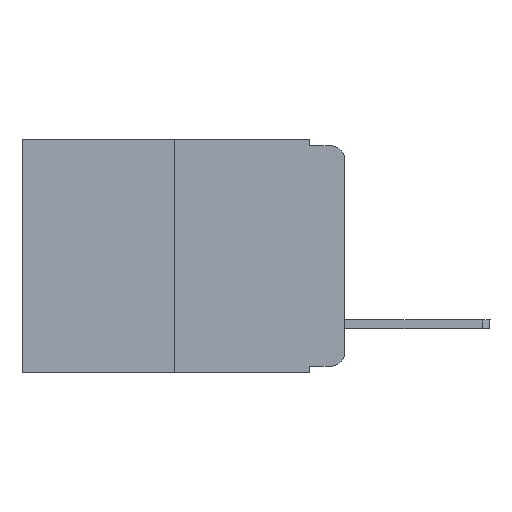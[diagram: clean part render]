
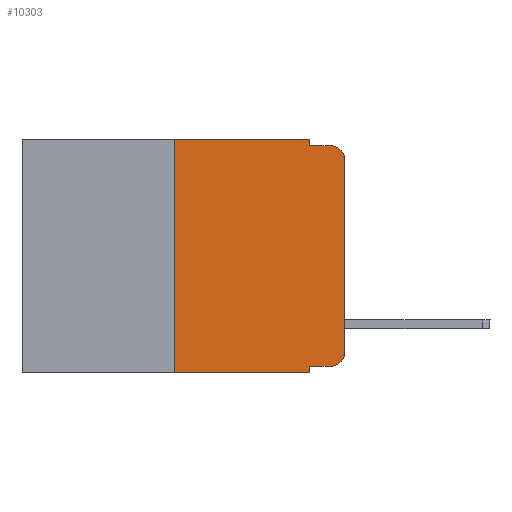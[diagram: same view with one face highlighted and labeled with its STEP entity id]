
A CAD part, left-side view. The second image highlights one B-rep face of the part: STEP entity #10303.
In plain terms, the highlighted planar face has unit normal (-1, 0, 0).
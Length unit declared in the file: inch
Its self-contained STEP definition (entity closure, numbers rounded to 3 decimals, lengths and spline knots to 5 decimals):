
#290 = VECTOR ( 'NONE', #5086, 39.37008 ) ;
#769 = CIRCLE ( 'NONE', #4019, 0.02 ) ;
#863 = ORIENTED_EDGE ( 'NONE', *, *, #11971, .T. ) ;
#1033 = ORIENTED_EDGE ( 'NONE', *, *, #11320, .F. ) ;
#1575 = VERTEX_POINT ( 'NONE', #14547 ) ;
#1820 = CARTESIAN_POINT ( 'NONE',  ( 0., 0.473, -0.343 ) ) ;
#1895 = LINE ( 'NONE', #1820, #14718 ) ;
#1922 = VERTEX_POINT ( 'NONE', #6890 ) ;
#2300 = EDGE_CURVE ( 'NONE', #1575, #3261, #2522, .T. ) ;
#2522 = LINE ( 'NONE', #7733, #9561 ) ;
#2606 = ORIENTED_EDGE ( 'NONE', *, *, #13235, .F. ) ;
#2616 = CARTESIAN_POINT ( 'NONE',  ( 0., 0.02, -0.313 ) ) ;
#2626 = LINE ( 'NONE', #11511, #290 ) ;
#2684 = EDGE_LOOP ( 'NONE', ( #15539, #863, #11656, #2606, #13786, #15054, #15966, #1033, #13511, #13650 ) ) ;
#2707 = CIRCLE ( 'NONE', #13351, 0.02 ) ;
#3261 = VERTEX_POINT ( 'NONE', #16416 ) ;
#3397 = VECTOR ( 'NONE', #13027, 39.37008 ) ;
#3613 = CARTESIAN_POINT ( 'NONE',  ( 0., 0., -0.03 ) ) ;
#3797 = PLANE ( 'NONE',  #15312 ) ;
#4019 = AXIS2_PLACEMENT_3D ( 'NONE', #2616, #7643, #11749 ) ;
#4460 = CARTESIAN_POINT ( 'NONE',  ( 0., 0.051, -0.343 ) ) ;
#4523 = VERTEX_POINT ( 'NONE', #6047 ) ;
#4895 = VERTEX_POINT ( 'NONE', #15977 ) ;
#5086 = DIRECTION ( 'NONE',  ( 0., 0., -1. ) ) ;
#5501 = EDGE_CURVE ( 'NONE', #10545, #11699, #16624, .T. ) ;
#5786 = VECTOR ( 'NONE', #5889, 39.37008 ) ;
#5889 = DIRECTION ( 'NONE',  ( 0., 0., -1. ) ) ;
#6047 = CARTESIAN_POINT ( 'NONE',  ( 0., 0.051, -0.01 ) ) ;
#6185 = CARTESIAN_POINT ( 'NONE',  ( 0., 0.25, 0. ) ) ;
#6357 = DIRECTION ( 'NONE',  ( 1., 0., 0. ) ) ;
#6890 = CARTESIAN_POINT ( 'NONE',  ( 0., 0., -0.313 ) ) ;
#7018 = DIRECTION ( 'NONE',  ( 0., -1., 0. ) ) ;
#7461 = CARTESIAN_POINT ( 'NONE',  ( 0., 0.051, -0.333 ) ) ;
#7544 = CARTESIAN_POINT ( 'NONE',  ( 0., 0.25, -0.343 ) ) ;
#7566 = LINE ( 'NONE', #6185, #9086 ) ;
#7643 = DIRECTION ( 'NONE',  ( -1., 0., 0. ) ) ;
#7645 = FACE_OUTER_BOUND ( 'NONE', #2684, .T. ) ;
#7733 = CARTESIAN_POINT ( 'NONE',  ( 0., 0.473, 0. ) ) ;
#8973 = EDGE_CURVE ( 'NONE', #11699, #1922, #769, .T. ) ;
#9086 = VECTOR ( 'NONE', #10475, 39.37008 ) ;
#9307 = CARTESIAN_POINT ( 'NONE',  ( 0., 0.051, -0.01 ) ) ;
#9561 = VECTOR ( 'NONE', #12958, 39.37008 ) ;
#9745 = EDGE_CURVE ( 'NONE', #16707, #12029, #1895, .T. ) ;
#10303 = ADVANCED_FACE ( 'NONE', ( #7645 ), #3797, .F. ) ;
#10361 = CARTESIAN_POINT ( 'NONE',  ( 0., 0.051, -0.333 ) ) ;
#10475 = DIRECTION ( 'NONE',  ( 0., 0., 1. ) ) ;
#10545 = VERTEX_POINT ( 'NONE', #7461 ) ;
#10773 = DIRECTION ( 'NONE',  ( 0., -1., 0. ) ) ;
#10793 = VECTOR ( 'NONE', #12101, 39.37008 ) ;
#10930 = LINE ( 'NONE', #9307, #14255 ) ;
#11320 = EDGE_CURVE ( 'NONE', #10545, #12029, #16822, .T. ) ;
#11468 = EDGE_CURVE ( 'NONE', #1922, #16649, #12011, .T. ) ;
#11511 = CARTESIAN_POINT ( 'NONE',  ( 0., 0.051, 0. ) ) ;
#11588 = DIRECTION ( 'NONE',  ( 0., 0., -1. ) ) ;
#11656 = ORIENTED_EDGE ( 'NONE', *, *, #15476, .F. ) ;
#11699 = VERTEX_POINT ( 'NONE', #13806 ) ;
#11749 = DIRECTION ( 'NONE',  ( 0., 0., -1. ) ) ;
#11971 = EDGE_CURVE ( 'NONE', #16649, #4895, #2707, .T. ) ;
#12011 = LINE ( 'NONE', #15859, #10793 ) ;
#12029 = VERTEX_POINT ( 'NONE', #4460 ) ;
#12101 = DIRECTION ( 'NONE',  ( 0., 0., 1. ) ) ;
#12869 = CARTESIAN_POINT ( 'NONE',  ( 0., 0.473, 0. ) ) ;
#12958 = DIRECTION ( 'NONE',  ( 0., -1., 0. ) ) ;
#13027 = DIRECTION ( 'NONE',  ( 0., -1., 0. ) ) ;
#13235 = EDGE_CURVE ( 'NONE', #3261, #4523, #2626, .T. ) ;
#13351 = AXIS2_PLACEMENT_3D ( 'NONE', #14986, #14910, #13697 ) ;
#13511 = ORIENTED_EDGE ( 'NONE', *, *, #5501, .T. ) ;
#13650 = ORIENTED_EDGE ( 'NONE', *, *, #8973, .T. ) ;
#13697 = DIRECTION ( 'NONE',  ( 0., 0., -1. ) ) ;
#13786 = ORIENTED_EDGE ( 'NONE', *, *, #2300, .F. ) ;
#13806 = CARTESIAN_POINT ( 'NONE',  ( 0., 0.02, -0.333 ) ) ;
#14255 = VECTOR ( 'NONE', #10773, 39.37008 ) ;
#14547 = CARTESIAN_POINT ( 'NONE',  ( 0., 0.25, 0. ) ) ;
#14718 = VECTOR ( 'NONE', #7018, 39.37008 ) ;
#14910 = DIRECTION ( 'NONE',  ( -1., 0., 0. ) ) ;
#14986 = CARTESIAN_POINT ( 'NONE',  ( 0., 0.02, -0.03 ) ) ;
#15054 = ORIENTED_EDGE ( 'NONE', *, *, #16208, .F. ) ;
#15312 = AXIS2_PLACEMENT_3D ( 'NONE', #12869, #6357, #11588 ) ;
#15476 = EDGE_CURVE ( 'NONE', #4523, #4895, #10930, .T. ) ;
#15539 = ORIENTED_EDGE ( 'NONE', *, *, #11468, .T. ) ;
#15859 = CARTESIAN_POINT ( 'NONE',  ( 0., 0., 0. ) ) ;
#15966 = ORIENTED_EDGE ( 'NONE', *, *, #9745, .T. ) ;
#15977 = CARTESIAN_POINT ( 'NONE',  ( 0., 0.02, -0.01 ) ) ;
#16208 = EDGE_CURVE ( 'NONE', #16707, #1575, #7566, .T. ) ;
#16416 = CARTESIAN_POINT ( 'NONE',  ( 0., 0.051, 0. ) ) ;
#16514 = CARTESIAN_POINT ( 'NONE',  ( 0., 0.051, 0. ) ) ;
#16624 = LINE ( 'NONE', #10361, #3397 ) ;
#16649 = VERTEX_POINT ( 'NONE', #3613 ) ;
#16707 = VERTEX_POINT ( 'NONE', #7544 ) ;
#16822 = LINE ( 'NONE', #16514, #5786 ) ;
